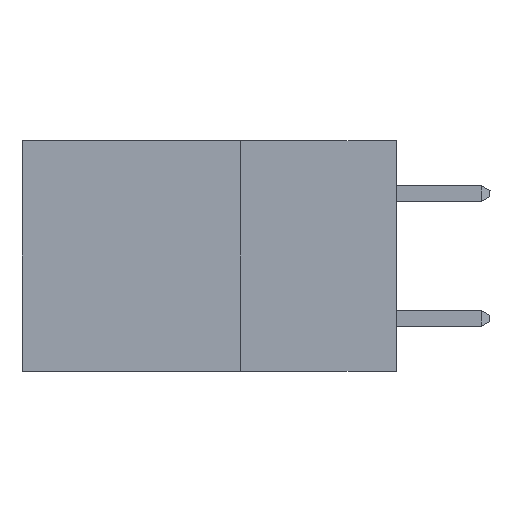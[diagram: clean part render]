
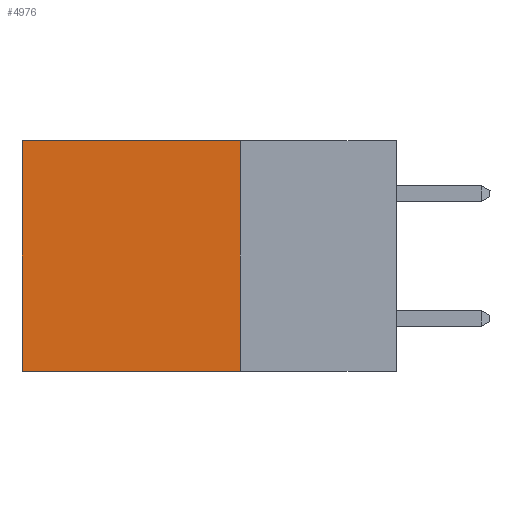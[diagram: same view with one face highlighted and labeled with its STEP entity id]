
A CAD part, left-side view. The second image highlights one B-rep face of the part: STEP entity #4976.
In plain terms, the highlighted planar face has unit normal (-1, 0, 0).
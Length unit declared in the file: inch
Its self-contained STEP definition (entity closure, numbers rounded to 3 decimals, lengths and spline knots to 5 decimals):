
#543 = DIRECTION ( 'NONE',  ( 0., 0., -1. ) ) ;
#608 = ORIENTED_EDGE ( 'NONE', *, *, #11826, .F. ) ;
#696 = VERTEX_POINT ( 'NONE', #2088 ) ;
#885 = CARTESIAN_POINT ( 'NONE',  ( 0.298, 0.25, -0.37 ) ) ;
#895 = DIRECTION ( 'NONE',  ( 1., 0., 0. ) ) ;
#1007 = VECTOR ( 'NONE', #3188, 39.37008 ) ;
#1092 = EDGE_LOOP ( 'NONE', ( #6686, #608, #8249, #6351 ) ) ;
#1322 = VECTOR ( 'NONE', #6982, 39.37008 ) ;
#1646 = CARTESIAN_POINT ( 'NONE',  ( 0.298, 0.25, -0.37 ) ) ;
#2088 = CARTESIAN_POINT ( 'NONE',  ( 0.298, 0.6, -0.37 ) ) ;
#3188 = DIRECTION ( 'NONE',  ( 0., 0., -1. ) ) ;
#3222 = VERTEX_POINT ( 'NONE', #885 ) ;
#3522 = DIRECTION ( 'NONE',  ( 0., 1., 0. ) ) ;
#4410 = VERTEX_POINT ( 'NONE', #8510 ) ;
#4421 = LINE ( 'NONE', #11917, #1322 ) ;
#4600 = EDGE_CURVE ( 'NONE', #6574, #696, #11107, .T. ) ;
#4976 = ADVANCED_FACE ( 'NONE', ( #5473 ), #12398, .F. ) ;
#4993 = CARTESIAN_POINT ( 'NONE',  ( 0.298, 0.6, 0. ) ) ;
#5473 = FACE_OUTER_BOUND ( 'NONE', #1092, .T. ) ;
#5712 = CARTESIAN_POINT ( 'NONE',  ( 0.298, 0.25, 0. ) ) ;
#5801 = DIRECTION ( 'NONE',  ( 0., 0., -1. ) ) ;
#6351 = ORIENTED_EDGE ( 'NONE', *, *, #8150, .T. ) ;
#6574 = VERTEX_POINT ( 'NONE', #4993 ) ;
#6686 = ORIENTED_EDGE ( 'NONE', *, *, #4600, .T. ) ;
#6982 = DIRECTION ( 'NONE',  ( 0., 1., 0. ) ) ;
#7117 = LINE ( 'NONE', #10339, #11520 ) ;
#7858 = AXIS2_PLACEMENT_3D ( 'NONE', #5712, #895, #5801 ) ;
#8150 = EDGE_CURVE ( 'NONE', #4410, #6574, #4421, .T. ) ;
#8249 = ORIENTED_EDGE ( 'NONE', *, *, #11994, .F. ) ;
#8510 = CARTESIAN_POINT ( 'NONE',  ( 0.298, 0.25, 0. ) ) ;
#8686 = VECTOR ( 'NONE', #3522, 39.37008 ) ;
#9921 = CARTESIAN_POINT ( 'NONE',  ( 0.298, 0.6, 0. ) ) ;
#10339 = CARTESIAN_POINT ( 'NONE',  ( 0.298, 0.25, 0. ) ) ;
#10924 = LINE ( 'NONE', #1646, #8686 ) ;
#11107 = LINE ( 'NONE', #9921, #1007 ) ;
#11520 = VECTOR ( 'NONE', #543, 39.37008 ) ;
#11826 = EDGE_CURVE ( 'NONE', #3222, #696, #10924, .T. ) ;
#11917 = CARTESIAN_POINT ( 'NONE',  ( 0.298, 0.25, 0. ) ) ;
#11994 = EDGE_CURVE ( 'NONE', #4410, #3222, #7117, .T. ) ;
#12398 = PLANE ( 'NONE',  #7858 ) ;
